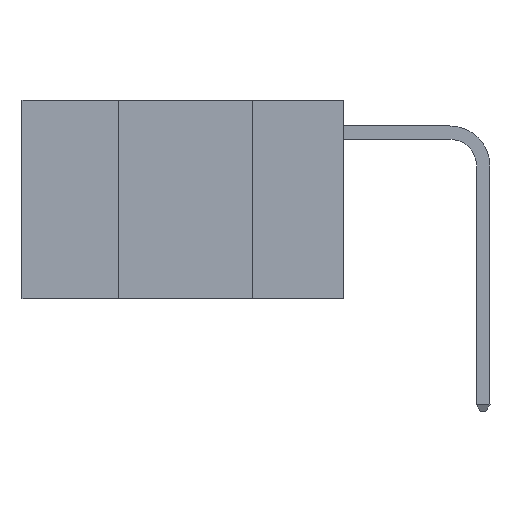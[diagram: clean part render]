
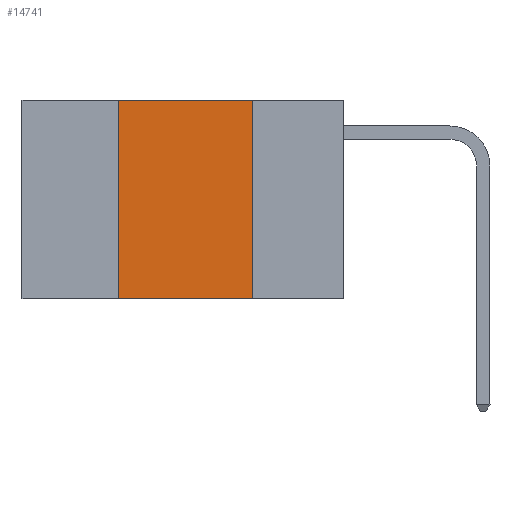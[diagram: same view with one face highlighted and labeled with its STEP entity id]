
A CAD part, left-side view. The second image highlights one B-rep face of the part: STEP entity #14741.
In plain terms, the highlighted planar face has unit normal (-1, 0, 0).
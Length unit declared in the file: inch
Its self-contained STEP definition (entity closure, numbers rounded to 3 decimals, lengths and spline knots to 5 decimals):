
#421 = PLANE ( 'NONE',  #22510 ) ;
#2174 = ORIENTED_EDGE ( 'NONE', *, *, #17322, .F. ) ;
#2906 = DIRECTION ( 'NONE',  ( 0., 0., 1. ) ) ;
#3190 = CARTESIAN_POINT ( 'NONE',  ( 0., 0.6, -0.37 ) ) ;
#4252 = ORIENTED_EDGE ( 'NONE', *, *, #12325, .F. ) ;
#4581 = VECTOR ( 'NONE', #2906, 39.37008 ) ;
#4805 = EDGE_CURVE ( 'NONE', #15760, #23233, #19341, .T. ) ;
#7712 = CARTESIAN_POINT ( 'NONE',  ( 0., 0.6, 0. ) ) ;
#8397 = ORIENTED_EDGE ( 'NONE', *, *, #20140, .F. ) ;
#8533 = EDGE_LOOP ( 'NONE', ( #2174, #4252, #8397, #18007 ) ) ;
#9690 = VERTEX_POINT ( 'NONE', #11960 ) ;
#10147 = VECTOR ( 'NONE', #17553, 39.37008 ) ;
#11832 = CARTESIAN_POINT ( 'NONE',  ( 0., 0.42, 0. ) ) ;
#11960 = CARTESIAN_POINT ( 'NONE',  ( 0., 0.42, 0. ) ) ;
#12121 = DIRECTION ( 'NONE',  ( 0., 0., -1. ) ) ;
#12236 = DIRECTION ( 'NONE',  ( 0., -1., 0. ) ) ;
#12325 = EDGE_CURVE ( 'NONE', #9690, #22368, #15427, .T. ) ;
#12774 = DIRECTION ( 'NONE',  ( 0., 0., -1. ) ) ;
#14530 = DIRECTION ( 'NONE',  ( 1., 0., 0. ) ) ;
#14741 = ADVANCED_FACE ( 'NONE', ( #21792 ), #421, .F. ) ;
#15427 = LINE ( 'NONE', #19376, #17563 ) ;
#15760 = VERTEX_POINT ( 'NONE', #19041 ) ;
#17322 = EDGE_CURVE ( 'NONE', #22368, #23233, #21351, .T. ) ;
#17553 = DIRECTION ( 'NONE',  ( 0., -1., 0. ) ) ;
#17563 = VECTOR ( 'NONE', #12236, 39.37008 ) ;
#18007 = ORIENTED_EDGE ( 'NONE', *, *, #4805, .T. ) ;
#18068 = VECTOR ( 'NONE', #12121, 39.37008 ) ;
#19041 = CARTESIAN_POINT ( 'NONE',  ( 0., 0.42, -0.37 ) ) ;
#19341 = LINE ( 'NONE', #3190, #10147 ) ;
#19376 = CARTESIAN_POINT ( 'NONE',  ( 0., 0.6, 0. ) ) ;
#20140 = EDGE_CURVE ( 'NONE', #15760, #9690, #23250, .T. ) ;
#21136 = CARTESIAN_POINT ( 'NONE',  ( 0., 0.17, 0. ) ) ;
#21351 = LINE ( 'NONE', #21136, #18068 ) ;
#21687 = CARTESIAN_POINT ( 'NONE',  ( 0., 0.17, 0. ) ) ;
#21792 = FACE_OUTER_BOUND ( 'NONE', #8533, .T. ) ;
#22086 = CARTESIAN_POINT ( 'NONE',  ( 0., 0.17, -0.37 ) ) ;
#22368 = VERTEX_POINT ( 'NONE', #21687 ) ;
#22510 = AXIS2_PLACEMENT_3D ( 'NONE', #7712, #14530, #12774 ) ;
#23233 = VERTEX_POINT ( 'NONE', #22086 ) ;
#23250 = LINE ( 'NONE', #11832, #4581 ) ;
